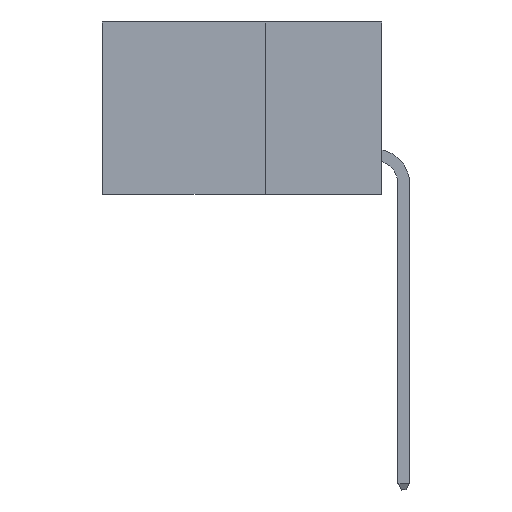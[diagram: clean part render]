
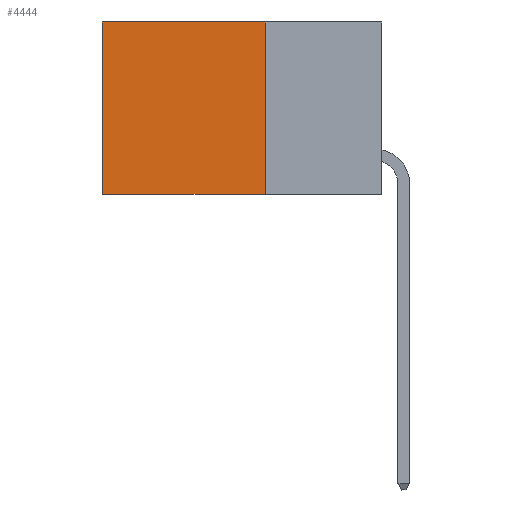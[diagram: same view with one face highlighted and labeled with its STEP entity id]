
A CAD part, left-side view. The second image highlights one B-rep face of the part: STEP entity #4444.
In plain terms, the highlighted planar face has unit normal (-1, 0, 0).
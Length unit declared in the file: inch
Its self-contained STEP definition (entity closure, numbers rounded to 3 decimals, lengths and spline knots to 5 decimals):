
#46 = ORIENTED_EDGE ( 'NONE', *, *, #10593, .F. ) ;
#598 = AXIS2_PLACEMENT_3D ( 'NONE', #14717, #12107, #27340 ) ;
#955 = EDGE_CURVE ( 'NONE', #13445, #2460, #25869, .T. ) ;
#1567 = DIRECTION ( 'NONE',  ( 0., 1., 0. ) ) ;
#1698 = CARTESIAN_POINT ( 'NONE',  ( 0.2875, 0.6, 0. ) ) ;
#1967 = CARTESIAN_POINT ( 'NONE',  ( 0.2875, 0.25, 0. ) ) ;
#2103 = PLANE ( 'NONE',  #598 ) ;
#2287 = VECTOR ( 'NONE', #16811, 39.37008 ) ;
#2460 = VERTEX_POINT ( 'NONE', #4048 ) ;
#4048 = CARTESIAN_POINT ( 'NONE',  ( 0.2875, 0.6, 0. ) ) ;
#4444 = ADVANCED_FACE ( 'NONE', ( #18691 ), #2103, .F. ) ;
#6568 = CARTESIAN_POINT ( 'NONE',  ( 0.2875, 0.25, -0.37 ) ) ;
#6571 = ORIENTED_EDGE ( 'NONE', *, *, #29255, .T. ) ;
#7762 = CARTESIAN_POINT ( 'NONE',  ( 0.2875, 0.25, 0. ) ) ;
#8605 = ORIENTED_EDGE ( 'NONE', *, *, #9724, .F. ) ;
#9045 = VECTOR ( 'NONE', #27954, 39.37008 ) ;
#9724 = EDGE_CURVE ( 'NONE', #13445, #28525, #22259, .T. ) ;
#10593 = EDGE_CURVE ( 'NONE', #28525, #17947, #19946, .T. ) ;
#12107 = DIRECTION ( 'NONE',  ( 1., 0., 0. ) ) ;
#13445 = VERTEX_POINT ( 'NONE', #7762 ) ;
#14125 = CARTESIAN_POINT ( 'NONE',  ( 0.2875, 0.25, -0.37 ) ) ;
#14717 = CARTESIAN_POINT ( 'NONE',  ( 0.2875, 0.25, 0. ) ) ;
#15430 = CARTESIAN_POINT ( 'NONE',  ( 0.2875, 0.25, 0. ) ) ;
#16811 = DIRECTION ( 'NONE',  ( 0., 0., -1. ) ) ;
#17947 = VERTEX_POINT ( 'NONE', #17977 ) ;
#17977 = CARTESIAN_POINT ( 'NONE',  ( 0.2875, 0.6, -0.37 ) ) ;
#18691 = FACE_OUTER_BOUND ( 'NONE', #27162, .T. ) ;
#19410 = DIRECTION ( 'NONE',  ( 0., 1., 0. ) ) ;
#19946 = LINE ( 'NONE', #6568, #30831 ) ;
#22074 = ORIENTED_EDGE ( 'NONE', *, *, #955, .T. ) ;
#22259 = LINE ( 'NONE', #15430, #9045 ) ;
#25475 = VECTOR ( 'NONE', #19410, 39.37008 ) ;
#25869 = LINE ( 'NONE', #1967, #25475 ) ;
#27162 = EDGE_LOOP ( 'NONE', ( #6571, #46, #8605, #22074 ) ) ;
#27340 = DIRECTION ( 'NONE',  ( 0., 0., -1. ) ) ;
#27954 = DIRECTION ( 'NONE',  ( 0., 0., -1. ) ) ;
#28525 = VERTEX_POINT ( 'NONE', #14125 ) ;
#28778 = LINE ( 'NONE', #1698, #2287 ) ;
#29255 = EDGE_CURVE ( 'NONE', #2460, #17947, #28778, .T. ) ;
#30831 = VECTOR ( 'NONE', #1567, 39.37008 ) ;
